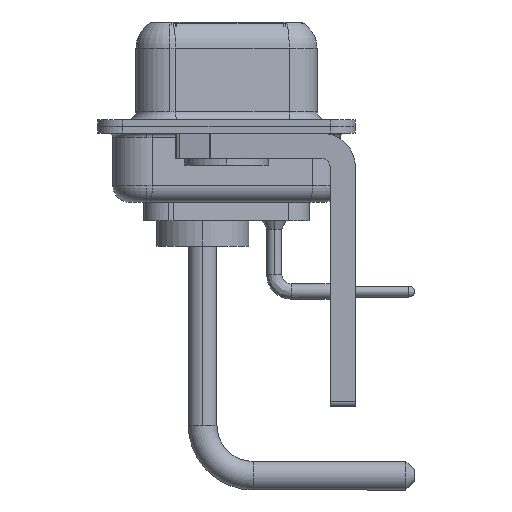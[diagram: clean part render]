
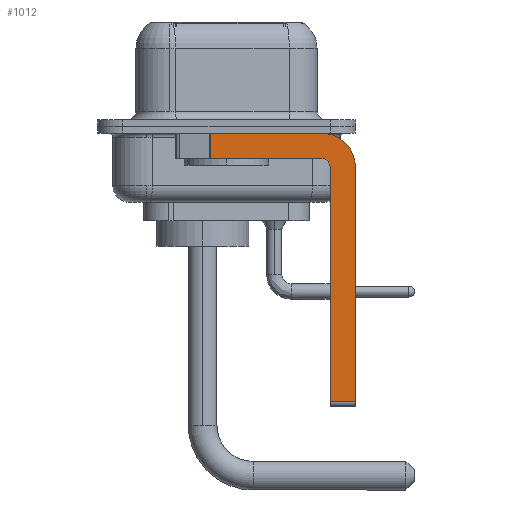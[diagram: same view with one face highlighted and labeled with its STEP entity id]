
A CAD part, left-side view. The second image highlights one B-rep face of the part: STEP entity #1012.
In plain terms, the highlighted planar face has unit normal (-1, 0, 0).
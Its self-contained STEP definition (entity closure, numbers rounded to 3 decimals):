
#655 = CIRCLE ( 'NONE', #9194, 0.5 ) ;
#1012 = ADVANCED_FACE ( 'NONE', ( #4078 ), #20882, .F. ) ;
#1024 = CARTESIAN_POINT ( 'NONE',  ( -2.9, 0.978, -1.9 ) ) ;
#1071 = CARTESIAN_POINT ( 'NONE',  ( -2.9, -5.65, -0.4 ) ) ;
#1084 = ORIENTED_EDGE ( 'NONE', *, *, #13524, .T. ) ;
#1288 = CARTESIAN_POINT ( 'NONE',  ( -2.9, -7.65, -2.4 ) ) ;
#1977 = LINE ( 'NONE', #12120, #9596 ) ;
#3695 = VERTEX_POINT ( 'NONE', #6721 ) ;
#3934 = EDGE_CURVE ( 'NONE', #3695, #14224, #13154, .T. ) ;
#4078 = FACE_OUTER_BOUND ( 'NONE', #21492, .T. ) ;
#4413 = DIRECTION ( 'NONE',  ( 0., 0., 1. ) ) ;
#4477 = VERTEX_POINT ( 'NONE', #1071 ) ;
#4601 = DIRECTION ( 'NONE',  ( -1., 0., 0. ) ) ;
#5064 = CARTESIAN_POINT ( 'NONE',  ( -2.9, -7.65, -2.4 ) ) ;
#5455 = ORIENTED_EDGE ( 'NONE', *, *, #3934, .T. ) ;
#5886 = CARTESIAN_POINT ( 'NONE',  ( -2.9, -5.65, -2.4 ) ) ;
#5986 = CARTESIAN_POINT ( 'NONE',  ( -2.9, -5.65, -1.9 ) ) ;
#6281 = DIRECTION ( 'NONE',  ( 0., 0., -1. ) ) ;
#6721 = CARTESIAN_POINT ( 'NONE',  ( -2.9, -6.15, -16.35 ) ) ;
#6918 = DIRECTION ( 'NONE',  ( 0., -1., 0. ) ) ;
#7028 = ORIENTED_EDGE ( 'NONE', *, *, #18615, .F. ) ;
#7379 = VECTOR ( 'NONE', #20204, 1000. ) ;
#7440 = DIRECTION ( 'NONE',  ( 1., 0., 0. ) ) ;
#7833 = EDGE_CURVE ( 'NONE', #18901, #14224, #20096, .T. ) ;
#8604 = EDGE_CURVE ( 'NONE', #17191, #15705, #17607, .T. ) ;
#8878 = LINE ( 'NONE', #11905, #18030 ) ;
#9194 = AXIS2_PLACEMENT_3D ( 'NONE', #16520, #4601, #21284 ) ;
#9306 = DIRECTION ( 'NONE',  ( 0., 0., -1. ) ) ;
#9423 = VECTOR ( 'NONE', #15163, 1000. ) ;
#9596 = VECTOR ( 'NONE', #4413, 1000. ) ;
#10657 = ORIENTED_EDGE ( 'NONE', *, *, #8604, .F. ) ;
#11124 = AXIS2_PLACEMENT_3D ( 'NONE', #15901, #7440, #9306 ) ;
#11818 = CARTESIAN_POINT ( 'NONE',  ( -2.9, -6.15, -2.4 ) ) ;
#11905 = CARTESIAN_POINT ( 'NONE',  ( -2.9, 3., -0.4 ) ) ;
#11978 = EDGE_CURVE ( 'NONE', #4477, #18901, #15457, .T. ) ;
#12120 = CARTESIAN_POINT ( 'NONE',  ( -2.9, -6.15, -16.6 ) ) ;
#12957 = VERTEX_POINT ( 'NONE', #19644 ) ;
#13154 = LINE ( 'NONE', #19807, #17461 ) ;
#13524 = EDGE_CURVE ( 'NONE', #12957, #15705, #16517, .T. ) ;
#13921 = CARTESIAN_POINT ( 'NONE',  ( -2.9, -7.65, -16.35 ) ) ;
#14101 = VECTOR ( 'NONE', #6281, 1000. ) ;
#14224 = VERTEX_POINT ( 'NONE', #13921 ) ;
#14347 = DIRECTION ( 'NONE',  ( 0., 0., -1. ) ) ;
#15163 = DIRECTION ( 'NONE',  ( 0., 1., 0. ) ) ;
#15457 = CIRCLE ( 'NONE', #18975, 2. ) ;
#15705 = VERTEX_POINT ( 'NONE', #16979 ) ;
#15901 = CARTESIAN_POINT ( 'NONE',  ( -2.9, -5.65, -2.4 ) ) ;
#16271 = DIRECTION ( 'NONE',  ( 0., -1., 0. ) ) ;
#16439 = DIRECTION ( 'NONE',  ( 1., 0., 0. ) ) ;
#16517 = LINE ( 'NONE', #1024, #14101 ) ;
#16520 = CARTESIAN_POINT ( 'NONE',  ( -2.9, -5.65, -2.4 ) ) ;
#16623 = EDGE_CURVE ( 'NONE', #12957, #4477, #8878, .T. ) ;
#16979 = CARTESIAN_POINT ( 'NONE',  ( -2.9, 0.978, -1.9 ) ) ;
#17191 = VERTEX_POINT ( 'NONE', #5986 ) ;
#17349 = ORIENTED_EDGE ( 'NONE', *, *, #17929, .F. ) ;
#17461 = VECTOR ( 'NONE', #16271, 1000. ) ;
#17607 = LINE ( 'NONE', #20228, #9423 ) ;
#17929 = EDGE_CURVE ( 'NONE', #18057, #17191, #655, .T. ) ;
#18030 = VECTOR ( 'NONE', #6918, 1000. ) ;
#18057 = VERTEX_POINT ( 'NONE', #11818 ) ;
#18460 = ORIENTED_EDGE ( 'NONE', *, *, #7833, .F. ) ;
#18615 = EDGE_CURVE ( 'NONE', #3695, #18057, #1977, .T. ) ;
#18901 = VERTEX_POINT ( 'NONE', #5064 ) ;
#18975 = AXIS2_PLACEMENT_3D ( 'NONE', #5886, #16439, #14347 ) ;
#19644 = CARTESIAN_POINT ( 'NONE',  ( -2.9, 0.978, -0.4 ) ) ;
#19803 = ORIENTED_EDGE ( 'NONE', *, *, #16623, .F. ) ;
#19807 = CARTESIAN_POINT ( 'NONE',  ( -2.9, -5.65, -16.35 ) ) ;
#20096 = LINE ( 'NONE', #1288, #7379 ) ;
#20204 = DIRECTION ( 'NONE',  ( 0., 0., -1. ) ) ;
#20228 = CARTESIAN_POINT ( 'NONE',  ( -2.9, -5.65, -1.9 ) ) ;
#20882 = PLANE ( 'NONE',  #11124 ) ;
#21284 = DIRECTION ( 'NONE',  ( 0., 0., 1. ) ) ;
#21492 = EDGE_LOOP ( 'NONE', ( #19803, #1084, #10657, #17349, #7028, #5455, #18460, #21543 ) ) ;
#21543 = ORIENTED_EDGE ( 'NONE', *, *, #11978, .F. ) ;
